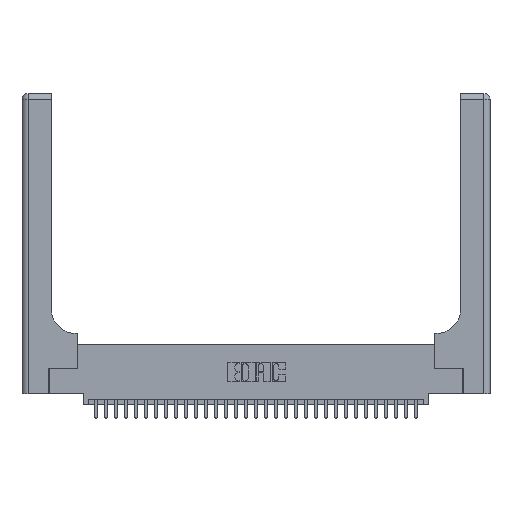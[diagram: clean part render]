
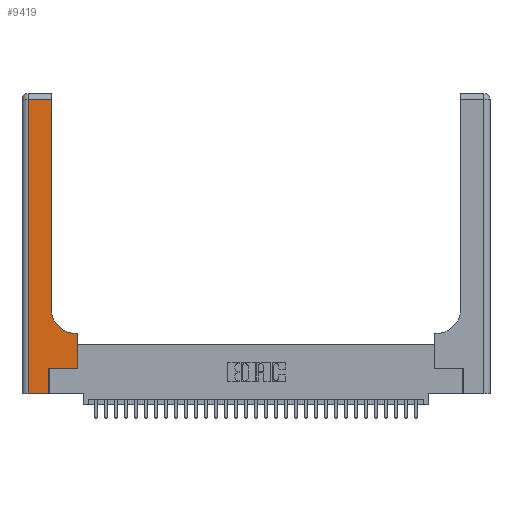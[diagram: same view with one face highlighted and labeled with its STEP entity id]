
A CAD part, top view. The second image highlights one B-rep face of the part: STEP entity #9419.
In plain terms, the highlighted planar face has unit normal (0, 0, 1).
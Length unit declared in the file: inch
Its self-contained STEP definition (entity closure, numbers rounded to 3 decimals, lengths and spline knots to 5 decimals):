
#492 = EDGE_LOOP ( 'NONE', ( #14434, #26442, #1699, #25041, #15012, #14636, #15042, #13859, #7571 ) ) ;
#781 = LINE ( 'NONE', #27811, #12745 ) ;
#792 = DIRECTION ( 'NONE',  ( -1., 0., 0. ) ) ;
#1291 = CARTESIAN_POINT ( 'NONE',  ( 0.5585, 0.6, 0.37 ) ) ;
#1699 = ORIENTED_EDGE ( 'NONE', *, *, #3974, .T. ) ;
#1927 = LINE ( 'NONE', #20630, #13882 ) ;
#2722 = EDGE_CURVE ( 'NONE', #27553, #4233, #29844, .T. ) ;
#3084 = DIRECTION ( 'NONE',  ( 0., 1., 0. ) ) ;
#3652 = EDGE_CURVE ( 'NONE', #3777, #27553, #29785, .T. ) ;
#3777 = VERTEX_POINT ( 'NONE', #27448 ) ;
#3905 = CIRCLE ( 'NONE', #11834, 0.25 ) ;
#3962 = VECTOR ( 'NONE', #24411, 39.37008 ) ;
#3974 = EDGE_CURVE ( 'NONE', #19283, #19107, #1927, .T. ) ;
#4032 = VECTOR ( 'NONE', #3084, 39.37008 ) ;
#4233 = VERTEX_POINT ( 'NONE', #1291 ) ;
#4650 = VECTOR ( 'NONE', #792, 39.37008 ) ;
#4658 = EDGE_CURVE ( 'NONE', #25766, #13322, #3905, .T. ) ;
#5047 = EDGE_CURVE ( 'NONE', #13322, #24709, #31986, .T. ) ;
#5535 = DIRECTION ( 'NONE',  ( 0., 0., -1. ) ) ;
#6091 = DIRECTION ( 'NONE',  ( 0., 1., 0. ) ) ;
#6958 = CARTESIAN_POINT ( 'NONE',  ( 0.269, 0.25, 0.37 ) ) ;
#7277 = FACE_OUTER_BOUND ( 'NONE', #492, .T. ) ;
#7571 = ORIENTED_EDGE ( 'NONE', *, *, #4658, .T. ) ;
#9419 = ADVANCED_FACE ( 'NONE', ( #7277 ), #21875, .F. ) ;
#9844 = DIRECTION ( 'NONE',  ( -1., 0., 0. ) ) ;
#10187 = EDGE_CURVE ( 'NONE', #24709, #19283, #781, .T. ) ;
#11834 = AXIS2_PLACEMENT_3D ( 'NONE', #20581, #5535, #23071 ) ;
#12125 = EDGE_CURVE ( 'NONE', #4233, #25766, #23104, .T. ) ;
#12745 = VECTOR ( 'NONE', #20357, 39.37008 ) ;
#13322 = VERTEX_POINT ( 'NONE', #27748 ) ;
#13859 = ORIENTED_EDGE ( 'NONE', *, *, #12125, .T. ) ;
#13882 = VECTOR ( 'NONE', #15650, 39.37008 ) ;
#13954 = CARTESIAN_POINT ( 'NONE',  ( 0., 0., 0.37 ) ) ;
#14434 = ORIENTED_EDGE ( 'NONE', *, *, #5047, .T. ) ;
#14636 = ORIENTED_EDGE ( 'NONE', *, *, #3652, .T. ) ;
#14659 = LINE ( 'NONE', #13954, #20467 ) ;
#15012 = ORIENTED_EDGE ( 'NONE', *, *, #17657, .T. ) ;
#15042 = ORIENTED_EDGE ( 'NONE', *, *, #2722, .T. ) ;
#15203 = LINE ( 'NONE', #23484, #21017 ) ;
#15650 = DIRECTION ( 'NONE',  ( 0., -1., 0. ) ) ;
#17119 = DIRECTION ( 'NONE',  ( 0., 1., 0. ) ) ;
#17657 = EDGE_CURVE ( 'NONE', #31716, #3777, #15203, .T. ) ;
#18257 = CARTESIAN_POINT ( 'NONE',  ( 0.5585, 0.25, 0.37 ) ) ;
#18954 = CARTESIAN_POINT ( 'NONE',  ( 0.2915, 2.94, 0.37 ) ) ;
#19107 = VERTEX_POINT ( 'NONE', #21577 ) ;
#19283 = VERTEX_POINT ( 'NONE', #29753 ) ;
#20357 = DIRECTION ( 'NONE',  ( -1., 0., 0. ) ) ;
#20467 = VECTOR ( 'NONE', #28780, 39.37008 ) ;
#20581 = CARTESIAN_POINT ( 'NONE',  ( 0.5415, 0.85, 0.37 ) ) ;
#20630 = CARTESIAN_POINT ( 'NONE',  ( 0.06, 3., 0.37 ) ) ;
#21017 = VECTOR ( 'NONE', #6091, 39.37008 ) ;
#21577 = CARTESIAN_POINT ( 'NONE',  ( 0.06, 0., 0.37 ) ) ;
#21875 = PLANE ( 'NONE',  #25434 ) ;
#22743 = CARTESIAN_POINT ( 'NONE',  ( 0.5585, 0.25, 0.37 ) ) ;
#23071 = DIRECTION ( 'NONE',  ( 1., 0., 0. ) ) ;
#23104 = LINE ( 'NONE', #23263, #4650 ) ;
#23263 = CARTESIAN_POINT ( 'NONE',  ( 0.2915, 0.6, 0.37 ) ) ;
#23484 = CARTESIAN_POINT ( 'NONE',  ( 0.269, 0., 0.37 ) ) ;
#24411 = DIRECTION ( 'NONE',  ( 1., 0., 0. ) ) ;
#24709 = VERTEX_POINT ( 'NONE', #18954 ) ;
#24720 = DIRECTION ( 'NONE',  ( 0., 0., -1. ) ) ;
#25041 = ORIENTED_EDGE ( 'NONE', *, *, #30666, .T. ) ;
#25434 = AXIS2_PLACEMENT_3D ( 'NONE', #26838, #24720, #9844 ) ;
#25456 = VECTOR ( 'NONE', #17119, 39.37008 ) ;
#25766 = VERTEX_POINT ( 'NONE', #28182 ) ;
#25830 = CARTESIAN_POINT ( 'NONE',  ( 0.269, 0., 0.37 ) ) ;
#26442 = ORIENTED_EDGE ( 'NONE', *, *, #10187, .T. ) ;
#26838 = CARTESIAN_POINT ( 'NONE',  ( 0., 3., 0.37 ) ) ;
#26945 = CARTESIAN_POINT ( 'NONE',  ( 0.2915, 3., 0.37 ) ) ;
#27448 = CARTESIAN_POINT ( 'NONE',  ( 0.269, 0.25, 0.37 ) ) ;
#27553 = VERTEX_POINT ( 'NONE', #22743 ) ;
#27748 = CARTESIAN_POINT ( 'NONE',  ( 0.2915, 0.85, 0.37 ) ) ;
#27811 = CARTESIAN_POINT ( 'NONE',  ( 0., 2.94, 0.37 ) ) ;
#28182 = CARTESIAN_POINT ( 'NONE',  ( 0.5415, 0.6, 0.37 ) ) ;
#28780 = DIRECTION ( 'NONE',  ( 1., 0., 0. ) ) ;
#29753 = CARTESIAN_POINT ( 'NONE',  ( 0.06, 2.94, 0.37 ) ) ;
#29785 = LINE ( 'NONE', #6958, #3962 ) ;
#29844 = LINE ( 'NONE', #18257, #4032 ) ;
#30666 = EDGE_CURVE ( 'NONE', #19107, #31716, #14659, .T. ) ;
#31716 = VERTEX_POINT ( 'NONE', #25830 ) ;
#31986 = LINE ( 'NONE', #26945, #25456 ) ;
